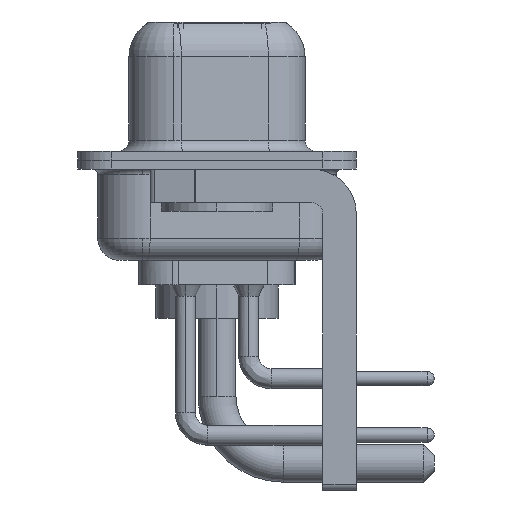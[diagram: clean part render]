
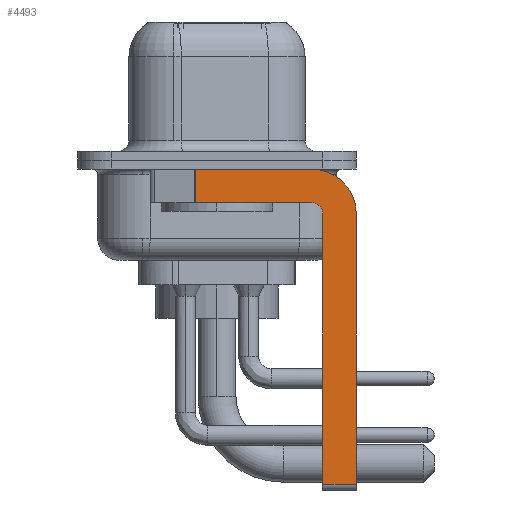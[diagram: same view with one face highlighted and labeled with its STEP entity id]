
A CAD part, left-side view. The second image highlights one B-rep face of the part: STEP entity #4493.
In plain terms, the highlighted planar face has unit normal (-1, 0, 0).
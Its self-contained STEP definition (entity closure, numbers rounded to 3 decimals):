
#226 = DIRECTION ( 'NONE',  ( 0., 0., 1. ) ) ;
#451 = EDGE_CURVE ( 'NONE', #6171, #3303, #19045, .T. ) ;
#461 = CARTESIAN_POINT ( 'NONE',  ( -2.9, -4.25, -2.4 ) ) ;
#855 = ORIENTED_EDGE ( 'NONE', *, *, #11545, .F. ) ;
#1144 = CARTESIAN_POINT ( 'NONE',  ( -2.9, -4.75, -14.55 ) ) ;
#1509 = EDGE_CURVE ( 'NONE', #11508, #5357, #4693, .T. ) ;
#1562 = CARTESIAN_POINT ( 'NONE',  ( -2.9, -4.25, -14.55 ) ) ;
#1775 = DIRECTION ( 'NONE',  ( 0., 0., -1. ) ) ;
#2390 = ORIENTED_EDGE ( 'NONE', *, *, #7839, .F. ) ;
#2755 = LINE ( 'NONE', #14380, #5165 ) ;
#2954 = CARTESIAN_POINT ( 'NONE',  ( -2.9, -4.75, -2.4 ) ) ;
#3013 = CARTESIAN_POINT ( 'NONE',  ( -2.9, -4.25, -2.4 ) ) ;
#3293 = DIRECTION ( 'NONE',  ( 0., 0., -1. ) ) ;
#3303 = VERTEX_POINT ( 'NONE', #13498 ) ;
#3328 = CARTESIAN_POINT ( 'NONE',  ( -2.9, -6.25, -14.55 ) ) ;
#3400 = EDGE_CURVE ( 'NONE', #11508, #6171, #18344, .T. ) ;
#3751 = ORIENTED_EDGE ( 'NONE', *, *, #5521, .F. ) ;
#4275 = DIRECTION ( 'NONE',  ( 1., 0., 0. ) ) ;
#4488 = LINE ( 'NONE', #1562, #18700 ) ;
#4493 = ADVANCED_FACE ( 'NONE', ( #5624 ), #8547, .F. ) ;
#4495 = ORIENTED_EDGE ( 'NONE', *, *, #3400, .F. ) ;
#4501 = LINE ( 'NONE', #4892, #7969 ) ;
#4573 = DIRECTION ( 'NONE',  ( 0., 0., -1. ) ) ;
#4693 = LINE ( 'NONE', #9169, #15985 ) ;
#4892 = CARTESIAN_POINT ( 'NONE',  ( -2.9, -4.75, -14.8 ) ) ;
#4973 = ORIENTED_EDGE ( 'NONE', *, *, #451, .F. ) ;
#4978 = VERTEX_POINT ( 'NONE', #5600 ) ;
#5165 = VECTOR ( 'NONE', #11790, 1000. ) ;
#5357 = VERTEX_POINT ( 'NONE', #12961 ) ;
#5521 = EDGE_CURVE ( 'NONE', #16305, #18333, #4501, .T. ) ;
#5600 = CARTESIAN_POINT ( 'NONE',  ( -2.9, -4.25, -1.9 ) ) ;
#5624 = FACE_OUTER_BOUND ( 'NONE', #11841, .T. ) ;
#6052 = CARTESIAN_POINT ( 'NONE',  ( -2.9, -4.25, -0.4 ) ) ;
#6171 = VERTEX_POINT ( 'NONE', #6052 ) ;
#6455 = ORIENTED_EDGE ( 'NONE', *, *, #1509, .T. ) ;
#6601 = DIRECTION ( 'NONE',  ( 0., -1., 0. ) ) ;
#6743 = CIRCLE ( 'NONE', #16341, 0.5 ) ;
#7112 = EDGE_CURVE ( 'NONE', #4978, #5357, #2755, .T. ) ;
#7839 = EDGE_CURVE ( 'NONE', #18333, #4978, #6743, .T. ) ;
#7969 = VECTOR ( 'NONE', #226, 1000. ) ;
#8060 = CARTESIAN_POINT ( 'NONE',  ( -2.9, 0.978, -0.4 ) ) ;
#8547 = PLANE ( 'NONE',  #15024 ) ;
#8929 = ORIENTED_EDGE ( 'NONE', *, *, #17358, .T. ) ;
#9169 = CARTESIAN_POINT ( 'NONE',  ( -2.9, 0.978, -1.9 ) ) ;
#9229 = DIRECTION ( 'NONE',  ( 0., 0., 1. ) ) ;
#10678 = CARTESIAN_POINT ( 'NONE',  ( -2.9, -6.25, -2.4 ) ) ;
#11508 = VERTEX_POINT ( 'NONE', #8060 ) ;
#11545 = EDGE_CURVE ( 'NONE', #3303, #18857, #12135, .T. ) ;
#11790 = DIRECTION ( 'NONE',  ( 0., 1., 0. ) ) ;
#11841 = EDGE_LOOP ( 'NONE', ( #4495, #6455, #15373, #2390, #3751, #8929, #855, #4973 ) ) ;
#12135 = LINE ( 'NONE', #10678, #16153 ) ;
#12419 = DIRECTION ( 'NONE',  ( -1., 0., 0. ) ) ;
#12961 = CARTESIAN_POINT ( 'NONE',  ( -2.9, 0.978, -1.9 ) ) ;
#13136 = DIRECTION ( 'NONE',  ( 0., -1., 0. ) ) ;
#13498 = CARTESIAN_POINT ( 'NONE',  ( -2.9, -6.25, -2.4 ) ) ;
#14380 = CARTESIAN_POINT ( 'NONE',  ( -2.9, -4.25, -1.9 ) ) ;
#14819 = CARTESIAN_POINT ( 'NONE',  ( -2.9, -4.25, -2.4 ) ) ;
#14994 = VECTOR ( 'NONE', #6601, 1000. ) ;
#15024 = AXIS2_PLACEMENT_3D ( 'NONE', #14819, #4275, #16001 ) ;
#15033 = DIRECTION ( 'NONE',  ( 1., 0., 0. ) ) ;
#15373 = ORIENTED_EDGE ( 'NONE', *, *, #7112, .F. ) ;
#15615 = AXIS2_PLACEMENT_3D ( 'NONE', #3013, #15033, #4573 ) ;
#15985 = VECTOR ( 'NONE', #1775, 1000. ) ;
#16001 = DIRECTION ( 'NONE',  ( 0., 0., -1. ) ) ;
#16153 = VECTOR ( 'NONE', #3293, 1000. ) ;
#16305 = VERTEX_POINT ( 'NONE', #1144 ) ;
#16341 = AXIS2_PLACEMENT_3D ( 'NONE', #461, #12419, #9229 ) ;
#17167 = CARTESIAN_POINT ( 'NONE',  ( -2.9, 3., -0.4 ) ) ;
#17358 = EDGE_CURVE ( 'NONE', #16305, #18857, #4488, .T. ) ;
#18333 = VERTEX_POINT ( 'NONE', #2954 ) ;
#18344 = LINE ( 'NONE', #17167, #14994 ) ;
#18700 = VECTOR ( 'NONE', #13136, 1000. ) ;
#18857 = VERTEX_POINT ( 'NONE', #3328 ) ;
#19045 = CIRCLE ( 'NONE', #15615, 2. ) ;
